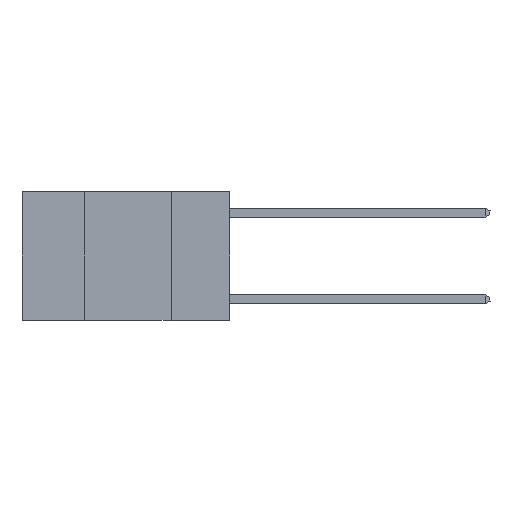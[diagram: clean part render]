
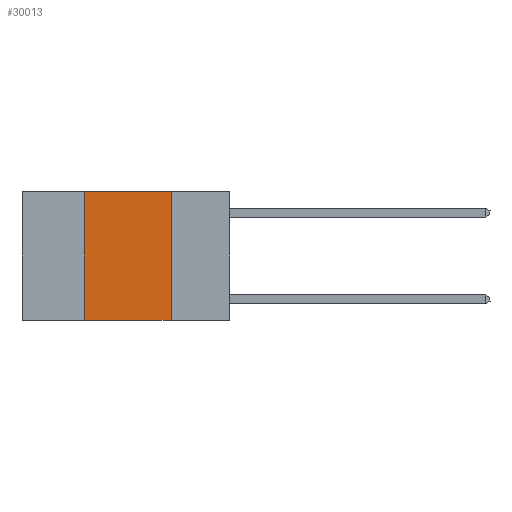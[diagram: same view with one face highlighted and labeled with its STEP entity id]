
A CAD part, left-side view. The second image highlights one B-rep face of the part: STEP entity #30013.
In plain terms, the highlighted planar face has unit normal (-1, 0, 0).
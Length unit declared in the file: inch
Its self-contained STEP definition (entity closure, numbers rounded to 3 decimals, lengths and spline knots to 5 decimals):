
#245 = EDGE_LOOP ( 'NONE', ( #13955, #15505, #29983, #4706 ) ) ;
#306 = FACE_OUTER_BOUND ( 'NONE', #245, .T. ) ;
#2181 = VECTOR ( 'NONE', #21454, 39.37008 ) ;
#2290 = CARTESIAN_POINT ( 'NONE',  ( 0., 0.42, 0. ) ) ;
#2883 = VECTOR ( 'NONE', #9864, 39.37008 ) ;
#4706 = ORIENTED_EDGE ( 'NONE', *, *, #5558, .T. ) ;
#5558 = EDGE_CURVE ( 'NONE', #10292, #7714, #20067, .T. ) ;
#7714 = VERTEX_POINT ( 'NONE', #21168 ) ;
#8177 = DIRECTION ( 'NONE',  ( 0., -1., 0. ) ) ;
#8564 = PLANE ( 'NONE',  #18904 ) ;
#8889 = CARTESIAN_POINT ( 'NONE',  ( 0., 0.17, 0. ) ) ;
#9864 = DIRECTION ( 'NONE',  ( 0., 0., 1. ) ) ;
#10292 = VERTEX_POINT ( 'NONE', #31096 ) ;
#10446 = VERTEX_POINT ( 'NONE', #2290 ) ;
#11037 = DIRECTION ( 'NONE',  ( 1., 0., 0. ) ) ;
#11186 = DIRECTION ( 'NONE',  ( 0., -1., 0. ) ) ;
#13554 = VECTOR ( 'NONE', #8177, 39.37008 ) ;
#13955 = ORIENTED_EDGE ( 'NONE', *, *, #22619, .F. ) ;
#15005 = EDGE_CURVE ( 'NONE', #10292, #10446, #28947, .T. ) ;
#15505 = ORIENTED_EDGE ( 'NONE', *, *, #20224, .F. ) ;
#18071 = VECTOR ( 'NONE', #11186, 39.37008 ) ;
#18490 = CARTESIAN_POINT ( 'NONE',  ( 0., 0.6, 0. ) ) ;
#18904 = AXIS2_PLACEMENT_3D ( 'NONE', #25714, #11037, #28152 ) ;
#19003 = CARTESIAN_POINT ( 'NONE',  ( 0., 0.17, 0. ) ) ;
#19060 = LINE ( 'NONE', #18490, #18071 ) ;
#20067 = LINE ( 'NONE', #27671, #13554 ) ;
#20224 = EDGE_CURVE ( 'NONE', #10446, #27995, #19060, .T. ) ;
#21168 = CARTESIAN_POINT ( 'NONE',  ( 0., 0.17, -0.37 ) ) ;
#21454 = DIRECTION ( 'NONE',  ( 0., 0., -1. ) ) ;
#21779 = LINE ( 'NONE', #19003, #2181 ) ;
#22087 = CARTESIAN_POINT ( 'NONE',  ( 0., 0.42, 0. ) ) ;
#22619 = EDGE_CURVE ( 'NONE', #27995, #7714, #21779, .T. ) ;
#25714 = CARTESIAN_POINT ( 'NONE',  ( 0., 0.6, 0. ) ) ;
#27671 = CARTESIAN_POINT ( 'NONE',  ( 0., 0.6, -0.37 ) ) ;
#27995 = VERTEX_POINT ( 'NONE', #8889 ) ;
#28152 = DIRECTION ( 'NONE',  ( 0., 0., -1. ) ) ;
#28947 = LINE ( 'NONE', #22087, #2883 ) ;
#29983 = ORIENTED_EDGE ( 'NONE', *, *, #15005, .F. ) ;
#30013 = ADVANCED_FACE ( 'NONE', ( #306 ), #8564, .F. ) ;
#31096 = CARTESIAN_POINT ( 'NONE',  ( 0., 0.42, -0.37 ) ) ;
